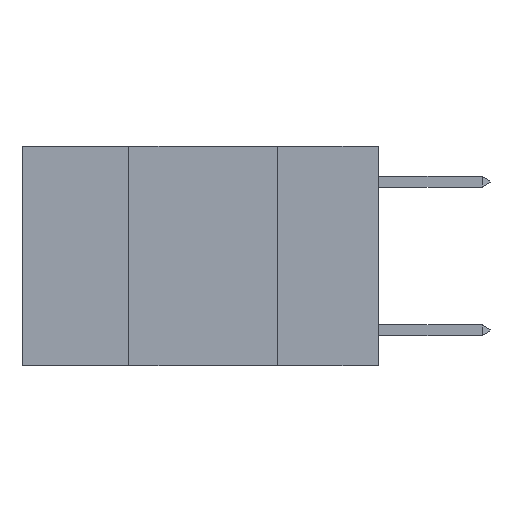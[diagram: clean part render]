
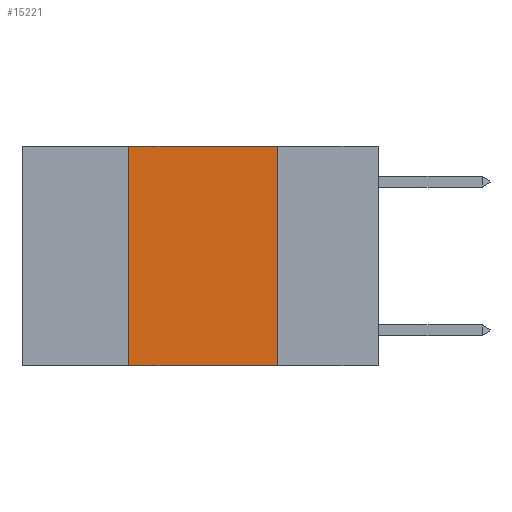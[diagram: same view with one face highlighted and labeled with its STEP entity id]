
A CAD part, left-side view. The second image highlights one B-rep face of the part: STEP entity #15221.
In plain terms, the highlighted planar face has unit normal (-1, 0, 0).
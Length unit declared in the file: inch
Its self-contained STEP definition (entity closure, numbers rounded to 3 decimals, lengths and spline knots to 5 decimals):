
#19 = CARTESIAN_POINT ( 'NONE',  ( 0., 0.42, 0. ) ) ;
#152 = VECTOR ( 'NONE', #2512, 39.37008 ) ;
#157 = VECTOR ( 'NONE', #3722, 39.37008 ) ;
#262 = LINE ( 'NONE', #2317, #152 ) ;
#479 = EDGE_CURVE ( 'NONE', #11879, #7483, #10107, .T. ) ;
#918 = DIRECTION ( 'NONE',  ( 0., 0., -1. ) ) ;
#977 = LINE ( 'NONE', #3816, #157 ) ;
#1778 = CARTESIAN_POINT ( 'NONE',  ( 0., 0.6, -0.37 ) ) ;
#2219 = VECTOR ( 'NONE', #12146, 39.37008 ) ;
#2317 = CARTESIAN_POINT ( 'NONE',  ( 0., 0.17, 0. ) ) ;
#2512 = DIRECTION ( 'NONE',  ( 0., 0., -1. ) ) ;
#3068 = EDGE_CURVE ( 'NONE', #8216, #3473, #262, .T. ) ;
#3473 = VERTEX_POINT ( 'NONE', #6212 ) ;
#3722 = DIRECTION ( 'NONE',  ( 0., -1., 0. ) ) ;
#3757 = ORIENTED_EDGE ( 'NONE', *, *, #16118, .T. ) ;
#3816 = CARTESIAN_POINT ( 'NONE',  ( 0., 0.6, 0. ) ) ;
#6212 = CARTESIAN_POINT ( 'NONE',  ( 0., 0.17, -0.37 ) ) ;
#6775 = EDGE_CURVE ( 'NONE', #7483, #8216, #977, .T. ) ;
#7258 = EDGE_LOOP ( 'NONE', ( #9494, #13431, #13608, #3757 ) ) ;
#7393 = PLANE ( 'NONE',  #15263 ) ;
#7483 = VERTEX_POINT ( 'NONE', #19 ) ;
#8216 = VERTEX_POINT ( 'NONE', #13190 ) ;
#8544 = CARTESIAN_POINT ( 'NONE',  ( 0., 0.42, -0.37 ) ) ;
#8715 = DIRECTION ( 'NONE',  ( 1., 0., 0. ) ) ;
#9494 = ORIENTED_EDGE ( 'NONE', *, *, #3068, .F. ) ;
#9903 = CARTESIAN_POINT ( 'NONE',  ( 0., 0.42, 0. ) ) ;
#10061 = VECTOR ( 'NONE', #10144, 39.37008 ) ;
#10107 = LINE ( 'NONE', #9903, #10061 ) ;
#10144 = DIRECTION ( 'NONE',  ( 0., 0., 1. ) ) ;
#11879 = VERTEX_POINT ( 'NONE', #8544 ) ;
#12146 = DIRECTION ( 'NONE',  ( 0., -1., 0. ) ) ;
#12166 = FACE_OUTER_BOUND ( 'NONE', #7258, .T. ) ;
#13190 = CARTESIAN_POINT ( 'NONE',  ( 0., 0.17, 0. ) ) ;
#13431 = ORIENTED_EDGE ( 'NONE', *, *, #6775, .F. ) ;
#13608 = ORIENTED_EDGE ( 'NONE', *, *, #479, .F. ) ;
#14936 = CARTESIAN_POINT ( 'NONE',  ( 0., 0.6, 0. ) ) ;
#15221 = ADVANCED_FACE ( 'NONE', ( #12166 ), #7393, .F. ) ;
#15263 = AXIS2_PLACEMENT_3D ( 'NONE', #14936, #8715, #918 ) ;
#15737 = LINE ( 'NONE', #1778, #2219 ) ;
#16118 = EDGE_CURVE ( 'NONE', #11879, #3473, #15737, .T. ) ;
